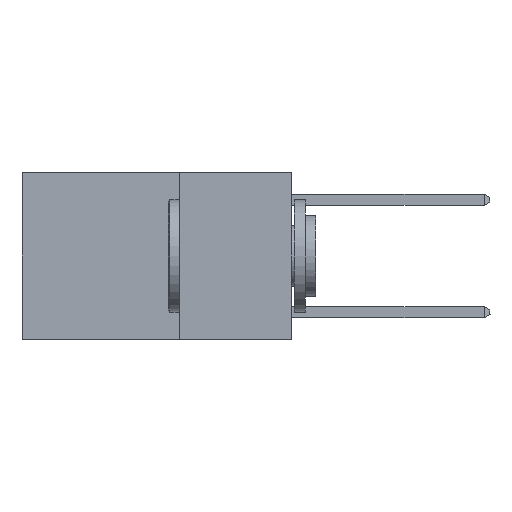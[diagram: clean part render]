
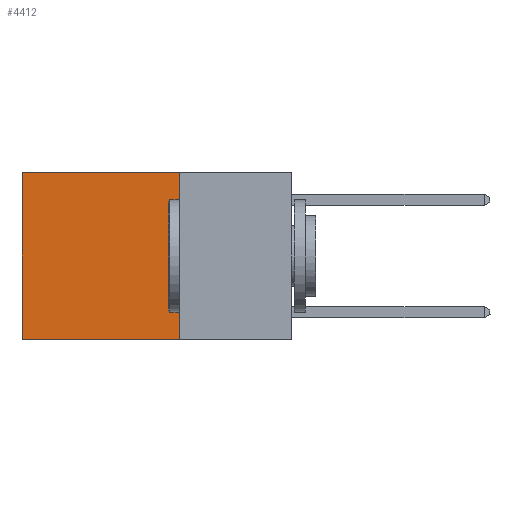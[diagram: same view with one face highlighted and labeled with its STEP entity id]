
A CAD part, left-side view. The second image highlights one B-rep face of the part: STEP entity #4412.
In plain terms, the highlighted planar face has unit normal (-1, 0, 0).
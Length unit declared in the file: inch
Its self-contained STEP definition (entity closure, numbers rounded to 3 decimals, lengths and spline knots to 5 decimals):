
#142 = FACE_OUTER_BOUND ( 'NONE', #9367, .T. ) ;
#222 = LINE ( 'NONE', #4662, #8219 ) ;
#666 = VECTOR ( 'NONE', #9699, 39.37008 ) ;
#850 = LINE ( 'NONE', #10558, #11185 ) ;
#1136 = ORIENTED_EDGE ( 'NONE', *, *, #6725, .T. ) ;
#1367 = CARTESIAN_POINT ( 'NONE',  ( 0.2625, 0.6, 0. ) ) ;
#1742 = VECTOR ( 'NONE', #8515, 39.37008 ) ;
#1790 = CARTESIAN_POINT ( 'NONE',  ( 0.2625, 0.25, -0.37 ) ) ;
#1872 = ORIENTED_EDGE ( 'NONE', *, *, #2965, .T. ) ;
#1932 = CARTESIAN_POINT ( 'NONE',  ( 0.2625, 0.25, 0. ) ) ;
#2653 = DIRECTION ( 'NONE',  ( 0., 0., -1. ) ) ;
#2965 = EDGE_CURVE ( 'NONE', #10637, #4772, #6667, .T. ) ;
#3016 = VERTEX_POINT ( 'NONE', #3208 ) ;
#3208 = CARTESIAN_POINT ( 'NONE',  ( 0.2625, 0.25, -0.37 ) ) ;
#4412 = ADVANCED_FACE ( 'NONE', ( #142 ), #7175, .F. ) ;
#4662 = CARTESIAN_POINT ( 'NONE',  ( 0.2625, 0.25, 0. ) ) ;
#4772 = VERTEX_POINT ( 'NONE', #5145 ) ;
#5145 = CARTESIAN_POINT ( 'NONE',  ( 0.2625, 0.6, -0.37 ) ) ;
#5443 = DIRECTION ( 'NONE',  ( 0., 0., -1. ) ) ;
#5531 = CARTESIAN_POINT ( 'NONE',  ( 0.2625, 0.25, 0. ) ) ;
#6657 = VERTEX_POINT ( 'NONE', #5531 ) ;
#6667 = LINE ( 'NONE', #1367, #1742 ) ;
#6725 = EDGE_CURVE ( 'NONE', #6657, #10637, #222, .T. ) ;
#7114 = EDGE_CURVE ( 'NONE', #3016, #4772, #8011, .T. ) ;
#7175 = PLANE ( 'NONE',  #7457 ) ;
#7446 = EDGE_CURVE ( 'NONE', #6657, #3016, #850, .T. ) ;
#7457 = AXIS2_PLACEMENT_3D ( 'NONE', #1932, #10664, #5443 ) ;
#8011 = LINE ( 'NONE', #1790, #666 ) ;
#8219 = VECTOR ( 'NONE', #10804, 39.37008 ) ;
#8389 = CARTESIAN_POINT ( 'NONE',  ( 0.2625, 0.6, 0. ) ) ;
#8515 = DIRECTION ( 'NONE',  ( 0., 0., -1. ) ) ;
#9367 = EDGE_LOOP ( 'NONE', ( #1872, #10329, #10016, #1136 ) ) ;
#9699 = DIRECTION ( 'NONE',  ( 0., 1., 0. ) ) ;
#10016 = ORIENTED_EDGE ( 'NONE', *, *, #7446, .F. ) ;
#10329 = ORIENTED_EDGE ( 'NONE', *, *, #7114, .F. ) ;
#10558 = CARTESIAN_POINT ( 'NONE',  ( 0.2625, 0.25, 0. ) ) ;
#10637 = VERTEX_POINT ( 'NONE', #8389 ) ;
#10664 = DIRECTION ( 'NONE',  ( 1., 0., 0. ) ) ;
#10804 = DIRECTION ( 'NONE',  ( 0., 1., 0. ) ) ;
#11185 = VECTOR ( 'NONE', #2653, 39.37008 ) ;
